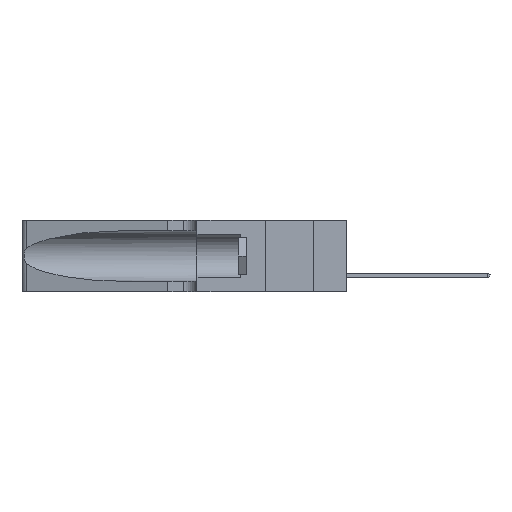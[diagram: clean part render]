
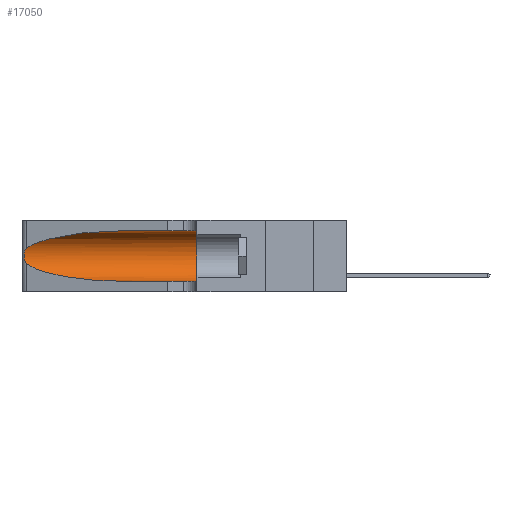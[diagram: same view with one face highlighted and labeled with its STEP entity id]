
A CAD part, left-side view. The second image highlights one B-rep face of the part: STEP entity #17050.
In plain terms, the highlighted cylindrical face has radius 3.308 mm (diameter 6.617 mm), a partial arc.
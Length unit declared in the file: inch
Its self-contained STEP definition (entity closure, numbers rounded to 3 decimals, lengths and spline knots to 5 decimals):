
#1788 = CARTESIAN_POINT ( 'NONE',  ( 0.25487, 1.22718, 0.14631 ) ) ;
#1842 = CYLINDRICAL_SURFACE ( 'NONE', #34959, 0.13025 ) ;
#2087 = CARTESIAN_POINT ( 'NONE',  ( 0.1305, 1.61858, 0.31525 ) ) ;
#2123 = CARTESIAN_POINT ( 'NONE',  ( 0.1305, 0.35, 0.185 ) ) ;
#2438 = CARTESIAN_POINT ( 'NONE',  ( 0.25854, 1.2359, 0.20912 ) ) ;
#2522 = CARTESIAN_POINT ( 'NONE',  ( 0.18966, 0.96281, 0.05475 ) ) ;
#3822 = EDGE_CURVE ( 'NONE', #8572, #32525, #15006, .T. ) ;
#4153 = B_SPLINE_CURVE_WITH_KNOTS ( 'NONE', 3,
 ( #28443, #30740, #17153, #5988, #2438, #34659, #11193, #31621, #22068, #21190, #22956, #29421, #19770, #10264 ),
 .UNSPECIFIED., .F., .F.,
 ( 4, 2, 2, 2, 2, 2, 4 ),
 ( 0., 0.00027, 0.00053, 0.00107, 0.0016, 0.00187, 0.00214 ),
 .UNSPECIFIED. ) ;
#5161 = DIRECTION ( 'NONE',  ( 0., 1., 0. ) ) ;
#5747 = CARTESIAN_POINT ( 'NONE',  ( 0.1305, 1.61858, 0.185 ) ) ;
#5908 = VERTEX_POINT ( 'NONE', #33109 ) ;
#5988 = CARTESIAN_POINT ( 'NONE',  ( 0.25787, 1.23484, 0.2124 ) ) ;
#6048 = CARTESIAN_POINT ( 'NONE',  ( 0.1305, 0.35, 0.05475 ) ) ;
#7655 = DIRECTION ( 'NONE',  ( 0., -1., 0. ) ) ;
#8273 = VECTOR ( 'NONE', #7655, 39.37008 ) ;
#8572 = VERTEX_POINT ( 'NONE', #27955 ) ;
#10162 = VERTEX_POINT ( 'NONE', #6048 ) ;
#10264 = CARTESIAN_POINT ( 'NONE',  ( 0.25487, 1.22718, 0.14631 ) ) ;
#10364 = VERTEX_POINT ( 'NONE', #1788 ) ;
#11193 = CARTESIAN_POINT ( 'NONE',  ( 0.26075, 1.23896, 0.19203 ) ) ;
#11263 = DIRECTION ( 'NONE',  ( 0., -1., 0. ) ) ;
#11503 = DIRECTION ( 'NONE',  ( 0., 0., -1. ) ) ;
#11593 = ORIENTED_EDGE ( 'NONE', *, *, #31983, .T. ) ;
#11694 = CARTESIAN_POINT ( 'NONE',  ( 0.1305, 0.72297, 0.31525 ) ) ;
#11893 = AXIS2_PLACEMENT_3D ( 'NONE', #2123, #5161, #15971 ) ;
#13045 = CARTESIAN_POINT ( 'NONE',  ( 0.25487, 1.22718, 0.14631 ) ) ;
#13824 = ORIENTED_EDGE ( 'NONE', *, *, #3822, .T. ) ;
#14780 = ORIENTED_EDGE ( 'NONE', *, *, #15041, .T. ) ;
#15006 =( BOUNDED_CURVE ( )  B_SPLINE_CURVE ( 3, ( #11694, #33334, #25096, #20123 ),
 .UNSPECIFIED., .F., .F. ) 
 B_SPLINE_CURVE_WITH_KNOTS ( ( 4, 4 ),
 ( 1.5708, 2.84003 ),
 .UNSPECIFIED. ) 
 CURVE ( )  GEOMETRIC_REPRESENTATION_ITEM ( )  RATIONAL_B_SPLINE_CURVE ( ( 1., 0.87, 0.87, 1. ) ) 
 REPRESENTATION_ITEM ( '' )  );
#15041 = EDGE_CURVE ( 'NONE', #32525, #10364, #4153, .T. ) ;
#15163 = ORIENTED_EDGE ( 'NONE', *, *, #34004, .T. ) ;
#15800 = CARTESIAN_POINT ( 'NONE',  ( 0.1305, 0.72297, 0.05475 ) ) ;
#15971 = DIRECTION ( 'NONE',  ( 0., 0., 1. ) ) ;
#16566 = ORIENTED_EDGE ( 'NONE', *, *, #31435, .F. ) ;
#17050 = ADVANCED_FACE ( 'NONE', ( #21278 ), #1842, .F. ) ;
#17153 = CARTESIAN_POINT ( 'NONE',  ( 0.25639, 1.23184, 0.21858 ) ) ;
#17629 = CARTESIAN_POINT ( 'NONE',  ( 0.1305, 1.61858, 0.05475 ) ) ;
#17761 = EDGE_LOOP ( 'NONE', ( #13824, #14780, #11593, #15163, #20462, #16566 ) ) ;
#19770 = CARTESIAN_POINT ( 'NONE',  ( 0.25555, 1.22993, 0.14849 ) ) ;
#20123 = CARTESIAN_POINT ( 'NONE',  ( 0.25487, 1.22718, 0.22369 ) ) ;
#20462 = ORIENTED_EDGE ( 'NONE', *, *, #27913, .F. ) ;
#21190 = CARTESIAN_POINT ( 'NONE',  ( 0.25856, 1.23593, 0.16098 ) ) ;
#21278 = FACE_OUTER_BOUND ( 'NONE', #17761, .T. ) ;
#22068 = CARTESIAN_POINT ( 'NONE',  ( 0.26017, 1.23833, 0.17102 ) ) ;
#22956 = CARTESIAN_POINT ( 'NONE',  ( 0.25789, 1.23486, 0.15765 ) ) ;
#23348 = DIRECTION ( 'NONE',  ( 0., -1., 0. ) ) ;
#23360 = VERTEX_POINT ( 'NONE', #35632 ) ;
#24927 =( BOUNDED_CURVE ( )  B_SPLINE_CURVE ( 3, ( #13045, #35597, #2522, #15800 ),
 .UNSPECIFIED., .F., .F. ) 
 B_SPLINE_CURVE_WITH_KNOTS ( ( 4, 4 ),
 ( 3.44316, 4.71239 ),
 .UNSPECIFIED. ) 
 CURVE ( )  GEOMETRIC_REPRESENTATION_ITEM ( )  RATIONAL_B_SPLINE_CURVE ( ( 1., 0.87, 0.87, 1. ) ) 
 REPRESENTATION_ITEM ( '' )  );
#25096 = CARTESIAN_POINT ( 'NONE',  ( 0.2373, 1.15595, 0.28018 ) ) ;
#25375 = VECTOR ( 'NONE', #23348, 39.37008 ) ;
#26732 = CIRCLE ( 'NONE', #11893, 0.13025 ) ;
#27913 = EDGE_CURVE ( 'NONE', #23360, #10162, #26732, .T. ) ;
#27955 = CARTESIAN_POINT ( 'NONE',  ( 0.1305, 0.72297, 0.31525 ) ) ;
#28443 = CARTESIAN_POINT ( 'NONE',  ( 0.25487, 1.22718, 0.22369 ) ) ;
#28614 = LINE ( 'NONE', #2087, #8273 ) ;
#29421 = CARTESIAN_POINT ( 'NONE',  ( 0.25639, 1.23186, 0.15144 ) ) ;
#30201 = LINE ( 'NONE', #17629, #25375 ) ;
#30740 = CARTESIAN_POINT ( 'NONE',  ( 0.25555, 1.22994, 0.2215 ) ) ;
#31435 = EDGE_CURVE ( 'NONE', #8572, #23360, #28614, .T. ) ;
#31621 = CARTESIAN_POINT ( 'NONE',  ( 0.26075, 1.23896, 0.178 ) ) ;
#31983 = EDGE_CURVE ( 'NONE', #10364, #5908, #24927, .T. ) ;
#32525 = VERTEX_POINT ( 'NONE', #35170 ) ;
#33109 = CARTESIAN_POINT ( 'NONE',  ( 0.1305, 0.72297, 0.05475 ) ) ;
#33334 = CARTESIAN_POINT ( 'NONE',  ( 0.18966, 0.96281, 0.31525 ) ) ;
#34004 = EDGE_CURVE ( 'NONE', #5908, #10162, #30201, .T. ) ;
#34659 = CARTESIAN_POINT ( 'NONE',  ( 0.26018, 1.23835, 0.19895 ) ) ;
#34959 = AXIS2_PLACEMENT_3D ( 'NONE', #5747, #11263, #11503 ) ;
#35170 = CARTESIAN_POINT ( 'NONE',  ( 0.25487, 1.22718, 0.22369 ) ) ;
#35597 = CARTESIAN_POINT ( 'NONE',  ( 0.2373, 1.15595, 0.08982 ) ) ;
#35632 = CARTESIAN_POINT ( 'NONE',  ( 0.1305, 0.35, 0.31525 ) ) ;
